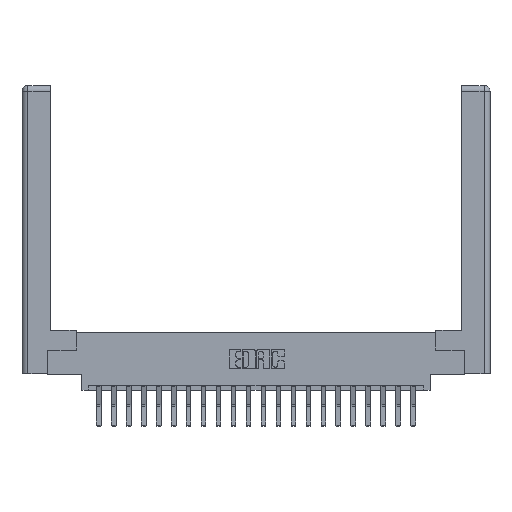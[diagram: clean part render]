
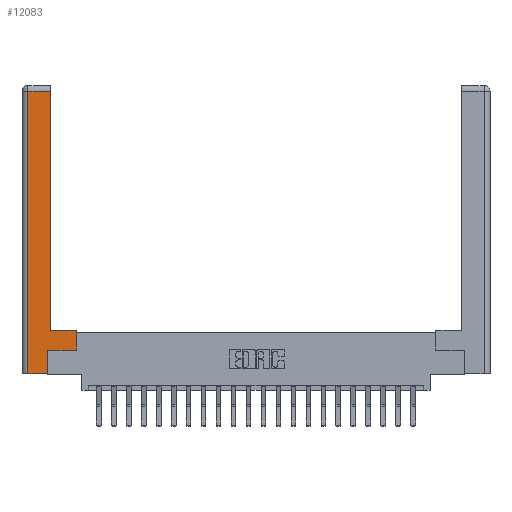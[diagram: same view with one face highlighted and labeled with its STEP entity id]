
A CAD part, top view. The second image highlights one B-rep face of the part: STEP entity #12083.
In plain terms, the highlighted planar face has unit normal (0, 0, 1).
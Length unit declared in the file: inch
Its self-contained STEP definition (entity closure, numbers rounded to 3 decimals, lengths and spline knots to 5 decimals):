
#222 = LINE ( 'NONE', #20637, #6771 ) ;
#835 = DIRECTION ( 'NONE',  ( -1., 0., 0. ) ) ;
#1233 = VECTOR ( 'NONE', #835, 39.37008 ) ;
#2031 = CARTESIAN_POINT ( 'NONE',  ( 0.565, 0.245, 0. ) ) ;
#2070 = ORIENTED_EDGE ( 'NONE', *, *, #7909, .T. ) ;
#2430 = VERTEX_POINT ( 'NONE', #12795 ) ;
#2829 = CARTESIAN_POINT ( 'NONE',  ( 0.265, 0., 0. ) ) ;
#3517 = CARTESIAN_POINT ( 'NONE',  ( 0.0615, 0., 0. ) ) ;
#3636 = DIRECTION ( 'NONE',  ( -1., 0., 0. ) ) ;
#3823 = CARTESIAN_POINT ( 'NONE',  ( 0.0615, 2.94, 0. ) ) ;
#3883 = ORIENTED_EDGE ( 'NONE', *, *, #4878, .T. ) ;
#3926 = VERTEX_POINT ( 'NONE', #2031 ) ;
#4678 = CARTESIAN_POINT ( 'NONE',  ( 0.265, 0., 0. ) ) ;
#4878 = EDGE_CURVE ( 'NONE', #3926, #5224, #8002, .T. ) ;
#4933 = DIRECTION ( 'NONE',  ( 0., 1., 0. ) ) ;
#5224 = VERTEX_POINT ( 'NONE', #21157 ) ;
#5405 = VERTEX_POINT ( 'NONE', #3517 ) ;
#5966 = CARTESIAN_POINT ( 'NONE',  ( 0.295, 0.45, 0. ) ) ;
#6227 = PLANE ( 'NONE',  #15455 ) ;
#6680 = LINE ( 'NONE', #5966, #1233 ) ;
#6754 = ORIENTED_EDGE ( 'NONE', *, *, #9351, .T. ) ;
#6771 = VECTOR ( 'NONE', #13846, 39.37008 ) ;
#7231 = ORIENTED_EDGE ( 'NONE', *, *, #16822, .T. ) ;
#7368 = CARTESIAN_POINT ( 'NONE',  ( 0.295, 2.94, 0. ) ) ;
#7434 = CARTESIAN_POINT ( 'NONE',  ( 0.295, 0.45, 0. ) ) ;
#7803 = EDGE_CURVE ( 'NONE', #2430, #3926, #222, .T. ) ;
#7892 = VECTOR ( 'NONE', #16703, 39.37008 ) ;
#7909 = EDGE_CURVE ( 'NONE', #20398, #2430, #17590, .T. ) ;
#8002 = LINE ( 'NONE', #19810, #15331 ) ;
#8432 = LINE ( 'NONE', #13185, #7892 ) ;
#9351 = EDGE_CURVE ( 'NONE', #16248, #5405, #11803, .T. ) ;
#9352 = EDGE_CURVE ( 'NONE', #5224, #18449, #6680, .T. ) ;
#9709 = CARTESIAN_POINT ( 'NONE',  ( 0.265, 0.245, 0. ) ) ;
#11803 = LINE ( 'NONE', #16077, #12088 ) ;
#12083 = ADVANCED_FACE ( 'NONE', ( #13348 ), #6227, .F. ) ;
#12088 = VECTOR ( 'NONE', #19547, 39.37008 ) ;
#12795 = CARTESIAN_POINT ( 'NONE',  ( 0.265, 0.245, 0. ) ) ;
#13066 = EDGE_CURVE ( 'NONE', #18449, #13694, #8432, .T. ) ;
#13185 = CARTESIAN_POINT ( 'NONE',  ( 0.295, 3., 0. ) ) ;
#13348 = FACE_OUTER_BOUND ( 'NONE', #19492, .T. ) ;
#13595 = DIRECTION ( 'NONE',  ( -1., 0., 0. ) ) ;
#13691 = LINE ( 'NONE', #4678, #20781 ) ;
#13694 = VERTEX_POINT ( 'NONE', #7368 ) ;
#13846 = DIRECTION ( 'NONE',  ( 1., 0., 0. ) ) ;
#13981 = CARTESIAN_POINT ( 'NONE',  ( 0.0615, 2.94, 0. ) ) ;
#14172 = ORIENTED_EDGE ( 'NONE', *, *, #21439, .T. ) ;
#14400 = ORIENTED_EDGE ( 'NONE', *, *, #7803, .T. ) ;
#15114 = LINE ( 'NONE', #13981, #16216 ) ;
#15331 = VECTOR ( 'NONE', #21474, 39.37008 ) ;
#15455 = AXIS2_PLACEMENT_3D ( 'NONE', #15505, #15572, #13595 ) ;
#15505 = CARTESIAN_POINT ( 'NONE',  ( 0., 0., 0. ) ) ;
#15572 = DIRECTION ( 'NONE',  ( 0., 0., -1. ) ) ;
#16077 = CARTESIAN_POINT ( 'NONE',  ( 0.0615, 0., 0. ) ) ;
#16216 = VECTOR ( 'NONE', #3636, 39.37008 ) ;
#16248 = VERTEX_POINT ( 'NONE', #3823 ) ;
#16703 = DIRECTION ( 'NONE',  ( 0., 1., 0. ) ) ;
#16822 = EDGE_CURVE ( 'NONE', #13694, #16248, #15114, .T. ) ;
#17590 = LINE ( 'NONE', #9709, #17873 ) ;
#17873 = VECTOR ( 'NONE', #4933, 39.37008 ) ;
#18449 = VERTEX_POINT ( 'NONE', #7434 ) ;
#19492 = EDGE_LOOP ( 'NONE', ( #21335, #7231, #6754, #14172, #2070, #14400, #3883, #19525 ) ) ;
#19525 = ORIENTED_EDGE ( 'NONE', *, *, #9352, .T. ) ;
#19547 = DIRECTION ( 'NONE',  ( 0., -1., 0. ) ) ;
#19810 = CARTESIAN_POINT ( 'NONE',  ( 0.565, 0.45, 0. ) ) ;
#20398 = VERTEX_POINT ( 'NONE', #2829 ) ;
#20637 = CARTESIAN_POINT ( 'NONE',  ( 0.565, 0.245, 0. ) ) ;
#20781 = VECTOR ( 'NONE', #22068, 39.37008 ) ;
#21157 = CARTESIAN_POINT ( 'NONE',  ( 0.565, 0.45, 0. ) ) ;
#21335 = ORIENTED_EDGE ( 'NONE', *, *, #13066, .T. ) ;
#21439 = EDGE_CURVE ( 'NONE', #5405, #20398, #13691, .T. ) ;
#21474 = DIRECTION ( 'NONE',  ( 0., 1., 0. ) ) ;
#22068 = DIRECTION ( 'NONE',  ( 1., 0., 0. ) ) ;
